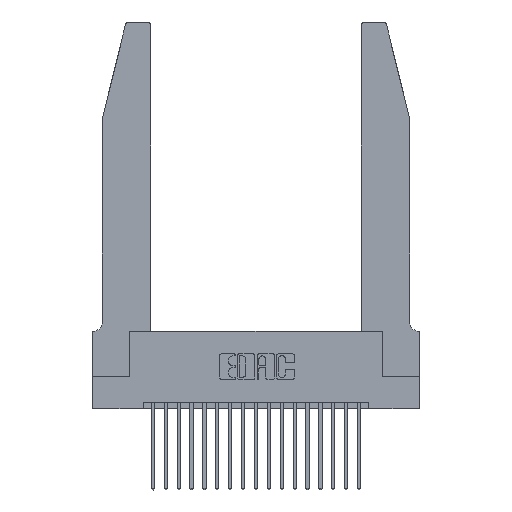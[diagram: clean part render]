
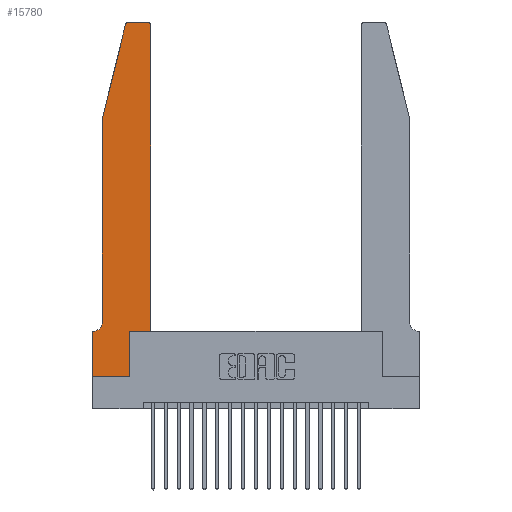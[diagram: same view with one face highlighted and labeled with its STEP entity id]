
A CAD part, top view. The second image highlights one B-rep face of the part: STEP entity #15780.
In plain terms, the highlighted planar face has unit normal (0, 0, 1).
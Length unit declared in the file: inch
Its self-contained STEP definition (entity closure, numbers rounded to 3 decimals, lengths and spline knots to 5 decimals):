
#209 = VERTEX_POINT ( 'NONE', #20982 ) ;
#267 = VECTOR ( 'NONE', #6221, 39.37008 ) ;
#345 = VECTOR ( 'NONE', #11088, 39.37008 ) ;
#807 = CARTESIAN_POINT ( 'NONE',  ( 0.25487, 2.72718, 0.37 ) ) ;
#907 = LINE ( 'NONE', #6142, #345 ) ;
#1163 = EDGE_CURVE ( 'NONE', #209, #5083, #13757, .T. ) ;
#1669 = EDGE_CURVE ( 'NONE', #9740, #2473, #3609, .T. ) ;
#1861 = AXIS2_PLACEMENT_3D ( 'NONE', #2218, #13811, #17149 ) ;
#2010 = DIRECTION ( 'NONE',  ( -1., 0., 0. ) ) ;
#2092 = DIRECTION ( 'NONE',  ( 1., 0., 0. ) ) ;
#2188 = EDGE_CURVE ( 'NONE', #2451, #19304, #6181, .T. ) ;
#2218 = CARTESIAN_POINT ( 'NONE',  ( 0., 0.35, 0.37 ) ) ;
#2295 = AXIS2_PLACEMENT_3D ( 'NONE', #17106, #18567, #2010 ) ;
#2395 = ORIENTED_EDGE ( 'NONE', *, *, #19130, .T. ) ;
#2451 = VERTEX_POINT ( 'NONE', #13008 ) ;
#2473 = VERTEX_POINT ( 'NONE', #14530 ) ;
#2491 = AXIS2_PLACEMENT_3D ( 'NONE', #14415, #17612, #17679 ) ;
#3104 = DIRECTION ( 'NONE',  ( -0.239, -0.971, 0. ) ) ;
#3269 = EDGE_CURVE ( 'NONE', #17361, #20508, #21337, .T. ) ;
#3547 = FACE_OUTER_BOUND ( 'NONE', #13606, .T. ) ;
#3609 = CIRCLE ( 'NONE', #9282, 0.03 ) ;
#4314 = LINE ( 'NONE', #17330, #13401 ) ;
#4802 = CARTESIAN_POINT ( 'NONE',  ( 0.0755, 0.42, 0.37 ) ) ;
#5083 = VERTEX_POINT ( 'NONE', #5819 ) ;
#5478 = CARTESIAN_POINT ( 'NONE',  ( 0., 0., 0.37 ) ) ;
#5819 = CARTESIAN_POINT ( 'NONE',  ( 0., 0.35, 0.37 ) ) ;
#6142 = CARTESIAN_POINT ( 'NONE',  ( 0., 0., 0.37 ) ) ;
#6181 = LINE ( 'NONE', #8773, #8779 ) ;
#6221 = DIRECTION ( 'NONE',  ( 0., -1., 0. ) ) ;
#7217 = DIRECTION ( 'NONE',  ( 0., 1., 0. ) ) ;
#7561 = ORIENTED_EDGE ( 'NONE', *, *, #20921, .T. ) ;
#7936 = CARTESIAN_POINT ( 'NONE',  ( 0.2865, 0.35, 0.37 ) ) ;
#8151 = CARTESIAN_POINT ( 'NONE',  ( 0.4505, 2.72, 0.37 ) ) ;
#8375 = LINE ( 'NONE', #20300, #21081 ) ;
#8534 = CIRCLE ( 'NONE', #2295, 0.07 ) ;
#8773 = CARTESIAN_POINT ( 'NONE',  ( 0.2865, 0.35, 0.37 ) ) ;
#8779 = VECTOR ( 'NONE', #18940, 39.37008 ) ;
#9051 = CARTESIAN_POINT ( 'NONE',  ( 0.4505, 0.35, 0.37 ) ) ;
#9282 = AXIS2_PLACEMENT_3D ( 'NONE', #19146, #15393, #2092 ) ;
#9366 = DIRECTION ( 'NONE',  ( -1., 0., 0. ) ) ;
#9590 = VERTEX_POINT ( 'NONE', #5478 ) ;
#9712 = CARTESIAN_POINT ( 'NONE',  ( 0.0755, 2., 0.37 ) ) ;
#9740 = VERTEX_POINT ( 'NONE', #8151 ) ;
#10451 = EDGE_CURVE ( 'NONE', #18573, #9740, #13627, .T. ) ;
#10622 = EDGE_CURVE ( 'NONE', #9590, #2451, #907, .T. ) ;
#10866 = CARTESIAN_POINT ( 'NONE',  ( 0.284, 2.75, 0.37 ) ) ;
#10935 = VECTOR ( 'NONE', #20505, 39.37008 ) ;
#11088 = DIRECTION ( 'NONE',  ( 1., 0., 0. ) ) ;
#11165 = CARTESIAN_POINT ( 'NONE',  ( 0.0755, 2., 0.37 ) ) ;
#11323 = VERTEX_POINT ( 'NONE', #4802 ) ;
#11544 = ORIENTED_EDGE ( 'NONE', *, *, #1669, .T. ) ;
#11890 = EDGE_CURVE ( 'NONE', #5083, #9590, #8375, .T. ) ;
#12312 = EDGE_CURVE ( 'NONE', #20508, #11323, #14343, .T. ) ;
#12383 = ORIENTED_EDGE ( 'NONE', *, *, #12312, .T. ) ;
#12474 = CARTESIAN_POINT ( 'NONE',  ( 0.2605, 2.75, 0.37 ) ) ;
#12543 = DIRECTION ( 'NONE',  ( 1., 0., 0. ) ) ;
#13008 = CARTESIAN_POINT ( 'NONE',  ( 0.2865, 0., 0.37 ) ) ;
#13193 = EDGE_CURVE ( 'NONE', #2473, #18608, #16378, .T. ) ;
#13401 = VECTOR ( 'NONE', #12543, 39.37008 ) ;
#13606 = EDGE_LOOP ( 'NONE', ( #19419, #2395, #16960, #12383, #16328, #21174, #18421, #14800, #19669, #7561, #15679, #11544 ) ) ;
#13627 = LINE ( 'NONE', #18030, #17803 ) ;
#13757 = LINE ( 'NONE', #19303, #16361 ) ;
#13811 = DIRECTION ( 'NONE',  ( 0., 0., 1. ) ) ;
#14343 = LINE ( 'NONE', #11165, #267 ) ;
#14415 = CARTESIAN_POINT ( 'NONE',  ( 0.284, 2.72, 0.37 ) ) ;
#14530 = CARTESIAN_POINT ( 'NONE',  ( 0.4205, 2.75, 0.37 ) ) ;
#14800 = ORIENTED_EDGE ( 'NONE', *, *, #10622, .T. ) ;
#15027 = DIRECTION ( 'NONE',  ( 0., -1., 0. ) ) ;
#15154 = EDGE_CURVE ( 'NONE', #11323, #209, #8534, .T. ) ;
#15393 = DIRECTION ( 'NONE',  ( 0., 0., 1. ) ) ;
#15679 = ORIENTED_EDGE ( 'NONE', *, *, #10451, .T. ) ;
#15780 = ADVANCED_FACE ( 'NONE', ( #3547 ), #18752, .T. ) ;
#16328 = ORIENTED_EDGE ( 'NONE', *, *, #15154, .T. ) ;
#16361 = VECTOR ( 'NONE', #9366, 39.37008 ) ;
#16378 = LINE ( 'NONE', #12474, #10935 ) ;
#16951 = VECTOR ( 'NONE', #3104, 39.37008 ) ;
#16960 = ORIENTED_EDGE ( 'NONE', *, *, #3269, .T. ) ;
#17106 = CARTESIAN_POINT ( 'NONE',  ( 0.0055, 0.42, 0.37 ) ) ;
#17149 = DIRECTION ( 'NONE',  ( 1., 0., 0. ) ) ;
#17330 = CARTESIAN_POINT ( 'NONE',  ( 0.4505, 0.35, 0.37 ) ) ;
#17361 = VERTEX_POINT ( 'NONE', #807 ) ;
#17612 = DIRECTION ( 'NONE',  ( 0., 0., 1. ) ) ;
#17679 = DIRECTION ( 'NONE',  ( 1., 0., 0. ) ) ;
#17803 = VECTOR ( 'NONE', #7217, 39.37008 ) ;
#18030 = CARTESIAN_POINT ( 'NONE',  ( 0.4505, 0.35, 0.37 ) ) ;
#18286 = CARTESIAN_POINT ( 'NONE',  ( 0.0755, 2., 0.37 ) ) ;
#18421 = ORIENTED_EDGE ( 'NONE', *, *, #11890, .T. ) ;
#18567 = DIRECTION ( 'NONE',  ( 0., 0., -1. ) ) ;
#18573 = VERTEX_POINT ( 'NONE', #9051 ) ;
#18608 = VERTEX_POINT ( 'NONE', #10866 ) ;
#18752 = PLANE ( 'NONE',  #1861 ) ;
#18940 = DIRECTION ( 'NONE',  ( 0., 1., 0. ) ) ;
#19130 = EDGE_CURVE ( 'NONE', #18608, #17361, #20731, .T. ) ;
#19146 = CARTESIAN_POINT ( 'NONE',  ( 0.4205, 2.72, 0.37 ) ) ;
#19303 = CARTESIAN_POINT ( 'NONE',  ( 0.0755, 0.35, 0.37 ) ) ;
#19304 = VERTEX_POINT ( 'NONE', #7936 ) ;
#19419 = ORIENTED_EDGE ( 'NONE', *, *, #13193, .T. ) ;
#19669 = ORIENTED_EDGE ( 'NONE', *, *, #2188, .T. ) ;
#20300 = CARTESIAN_POINT ( 'NONE',  ( 0., 0., 0.37 ) ) ;
#20505 = DIRECTION ( 'NONE',  ( -1., 0., 0. ) ) ;
#20508 = VERTEX_POINT ( 'NONE', #18286 ) ;
#20731 = CIRCLE ( 'NONE', #2491, 0.03 ) ;
#20921 = EDGE_CURVE ( 'NONE', #19304, #18573, #4314, .T. ) ;
#20982 = CARTESIAN_POINT ( 'NONE',  ( 0.0055, 0.35, 0.37 ) ) ;
#21081 = VECTOR ( 'NONE', #15027, 39.37008 ) ;
#21174 = ORIENTED_EDGE ( 'NONE', *, *, #1163, .T. ) ;
#21337 = LINE ( 'NONE', #9712, #16951 ) ;
